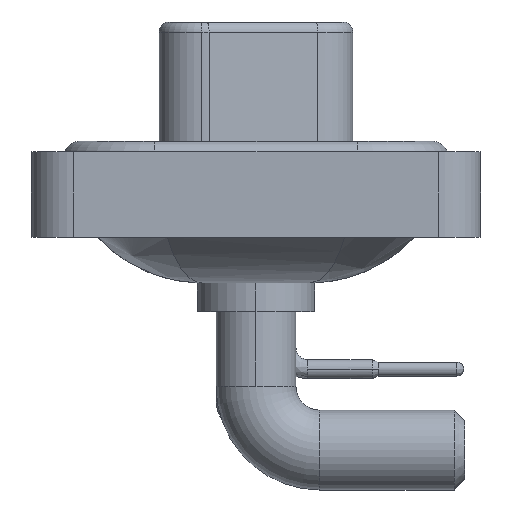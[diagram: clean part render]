
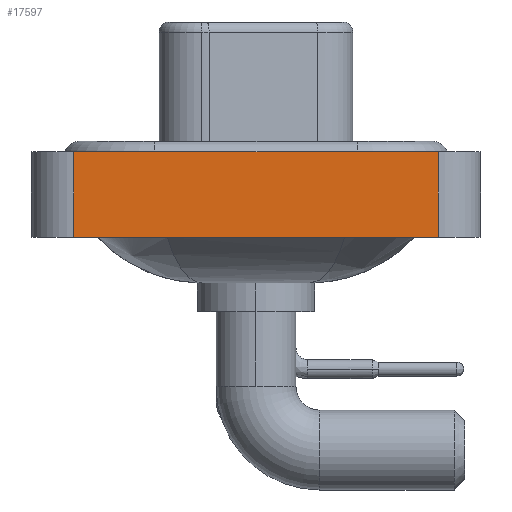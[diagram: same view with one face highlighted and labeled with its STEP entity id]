
A CAD part, left-side view. The second image highlights one B-rep face of the part: STEP entity #17597.
In plain terms, the highlighted planar face has unit normal (-1, 0, 0).
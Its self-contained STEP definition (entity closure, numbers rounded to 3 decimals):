
#2176 = CARTESIAN_POINT ( 'NONE',  ( -7.3, -8.55, 0.4 ) ) ;
#2870 = LINE ( 'NONE', #8462, #20082 ) ;
#3393 = CARTESIAN_POINT ( 'NONE',  ( -7.3, -8.55, -3.6 ) ) ;
#3688 = EDGE_CURVE ( 'NONE', #7970, #12783, #20418, .T. ) ;
#4459 = DIRECTION ( 'NONE',  ( -1., 0., 0. ) ) ;
#4573 = DIRECTION ( 'NONE',  ( 0., 0., 1. ) ) ;
#6287 = CARTESIAN_POINT ( 'NONE',  ( -7.3, 8.55, 0.4 ) ) ;
#7592 = ORIENTED_EDGE ( 'NONE', *, *, #19329, .T. ) ;
#7970 = VERTEX_POINT ( 'NONE', #20284 ) ;
#8462 = CARTESIAN_POINT ( 'NONE',  ( -7.3, -8.55, -3.6 ) ) ;
#8971 = EDGE_LOOP ( 'NONE', ( #14893, #23788, #14758, #7592 ) ) ;
#9210 = VERTEX_POINT ( 'NONE', #17563 ) ;
#9392 = DIRECTION ( 'NONE',  ( 0., 0., 1. ) ) ;
#10997 = CARTESIAN_POINT ( 'NONE',  ( -7.3, -8.55, 0.4 ) ) ;
#11175 = EDGE_CURVE ( 'NONE', #9210, #21632, #11631, .T. ) ;
#11439 = AXIS2_PLACEMENT_3D ( 'NONE', #17500, #4459, #4573 ) ;
#11631 = LINE ( 'NONE', #13498, #23414 ) ;
#12783 = VERTEX_POINT ( 'NONE', #10997 ) ;
#13498 = CARTESIAN_POINT ( 'NONE',  ( -7.3, 8.55, -3.6 ) ) ;
#13753 = PLANE ( 'NONE',  #11439 ) ;
#14060 = DIRECTION ( 'NONE',  ( 0., -1., 0. ) ) ;
#14758 = ORIENTED_EDGE ( 'NONE', *, *, #11175, .F. ) ;
#14893 = ORIENTED_EDGE ( 'NONE', *, *, #3688, .T. ) ;
#15730 = EDGE_CURVE ( 'NONE', #21632, #12783, #19180, .T. ) ;
#17500 = CARTESIAN_POINT ( 'NONE',  ( -7.3, -8.55, -3.6 ) ) ;
#17563 = CARTESIAN_POINT ( 'NONE',  ( -7.3, 8.55, -3.6 ) ) ;
#17597 = ADVANCED_FACE ( 'NONE', ( #21618 ), #13753, .T. ) ;
#19003 = VECTOR ( 'NONE', #21806, 1000. ) ;
#19180 = LINE ( 'NONE', #2176, #23297 ) ;
#19329 = EDGE_CURVE ( 'NONE', #9210, #7970, #2870, .T. ) ;
#19426 = DIRECTION ( 'NONE',  ( 0., -1., 0. ) ) ;
#20082 = VECTOR ( 'NONE', #14060, 1000. ) ;
#20284 = CARTESIAN_POINT ( 'NONE',  ( -7.3, -8.55, -3.6 ) ) ;
#20418 = LINE ( 'NONE', #3393, #19003 ) ;
#21618 = FACE_OUTER_BOUND ( 'NONE', #8971, .T. ) ;
#21632 = VERTEX_POINT ( 'NONE', #6287 ) ;
#21806 = DIRECTION ( 'NONE',  ( 0., 0., 1. ) ) ;
#23297 = VECTOR ( 'NONE', #19426, 1000. ) ;
#23414 = VECTOR ( 'NONE', #9392, 1000. ) ;
#23788 = ORIENTED_EDGE ( 'NONE', *, *, #15730, .F. ) ;
